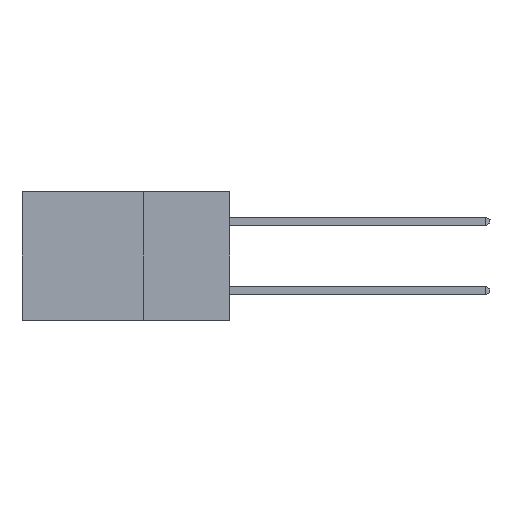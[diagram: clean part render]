
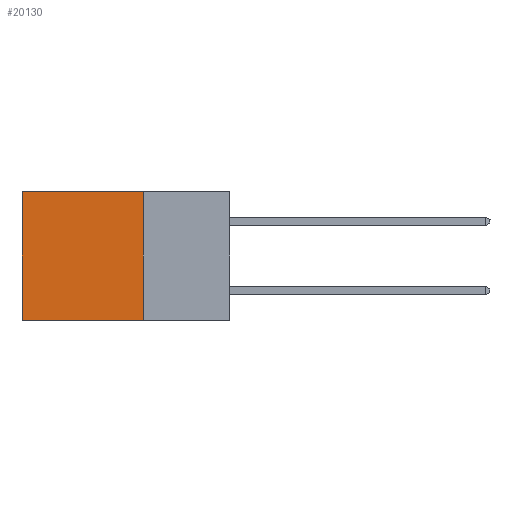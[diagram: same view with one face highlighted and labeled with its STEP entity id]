
A CAD part, left-side view. The second image highlights one B-rep face of the part: STEP entity #20130.
In plain terms, the highlighted planar face has unit normal (-1, 0, 0).
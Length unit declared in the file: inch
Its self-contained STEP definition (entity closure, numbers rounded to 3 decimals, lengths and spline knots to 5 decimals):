
#407 = CARTESIAN_POINT ( 'NONE',  ( 0.298, 0.25, 0. ) ) ;
#704 = DIRECTION ( 'NONE',  ( 0., 0., -1. ) ) ;
#1175 = DIRECTION ( 'NONE',  ( 0., 1., 0. ) ) ;
#1627 = CARTESIAN_POINT ( 'NONE',  ( 0.298, 0.25, 0. ) ) ;
#1784 = CARTESIAN_POINT ( 'NONE',  ( 0.298, 0.6, -0.37 ) ) ;
#2956 = ORIENTED_EDGE ( 'NONE', *, *, #22130, .T. ) ;
#3344 = EDGE_CURVE ( 'NONE', #9638, #10488, #16433, .T. ) ;
#4400 = VECTOR ( 'NONE', #1175, 39.37008 ) ;
#5096 = VECTOR ( 'NONE', #22771, 39.37008 ) ;
#7053 = VECTOR ( 'NONE', #19079, 39.37008 ) ;
#8631 = CARTESIAN_POINT ( 'NONE',  ( 0.298, 0.25, -0.37 ) ) ;
#9638 = VERTEX_POINT ( 'NONE', #17657 ) ;
#9828 = CARTESIAN_POINT ( 'NONE',  ( 0.298, 0.25, 0. ) ) ;
#10090 = VERTEX_POINT ( 'NONE', #14506 ) ;
#10157 = CARTESIAN_POINT ( 'NONE',  ( 0.298, 0.6, 0. ) ) ;
#10469 = VERTEX_POINT ( 'NONE', #1627 ) ;
#10488 = VERTEX_POINT ( 'NONE', #1784 ) ;
#10912 = EDGE_LOOP ( 'NONE', ( #18498, #12852, #22777, #2956 ) ) ;
#11089 = EDGE_CURVE ( 'NONE', #10469, #9638, #15024, .T. ) ;
#12510 = EDGE_CURVE ( 'NONE', #10090, #10488, #17011, .T. ) ;
#12852 = ORIENTED_EDGE ( 'NONE', *, *, #3344, .F. ) ;
#13844 = LINE ( 'NONE', #16950, #4400 ) ;
#14506 = CARTESIAN_POINT ( 'NONE',  ( 0.298, 0.6, 0. ) ) ;
#14739 = AXIS2_PLACEMENT_3D ( 'NONE', #407, #16304, #16369 ) ;
#15024 = LINE ( 'NONE', #9828, #20801 ) ;
#16304 = DIRECTION ( 'NONE',  ( 1., 0., 0. ) ) ;
#16369 = DIRECTION ( 'NONE',  ( 0., 0., -1. ) ) ;
#16433 = LINE ( 'NONE', #8631, #5096 ) ;
#16950 = CARTESIAN_POINT ( 'NONE',  ( 0.298, 0.25, 0. ) ) ;
#17011 = LINE ( 'NONE', #10157, #7053 ) ;
#17657 = CARTESIAN_POINT ( 'NONE',  ( 0.298, 0.25, -0.37 ) ) ;
#18498 = ORIENTED_EDGE ( 'NONE', *, *, #12510, .T. ) ;
#19079 = DIRECTION ( 'NONE',  ( 0., 0., -1. ) ) ;
#20130 = ADVANCED_FACE ( 'NONE', ( #20522 ), #21725, .F. ) ;
#20522 = FACE_OUTER_BOUND ( 'NONE', #10912, .T. ) ;
#20801 = VECTOR ( 'NONE', #704, 39.37008 ) ;
#21725 = PLANE ( 'NONE',  #14739 ) ;
#22130 = EDGE_CURVE ( 'NONE', #10469, #10090, #13844, .T. ) ;
#22771 = DIRECTION ( 'NONE',  ( 0., 1., 0. ) ) ;
#22777 = ORIENTED_EDGE ( 'NONE', *, *, #11089, .F. ) ;
